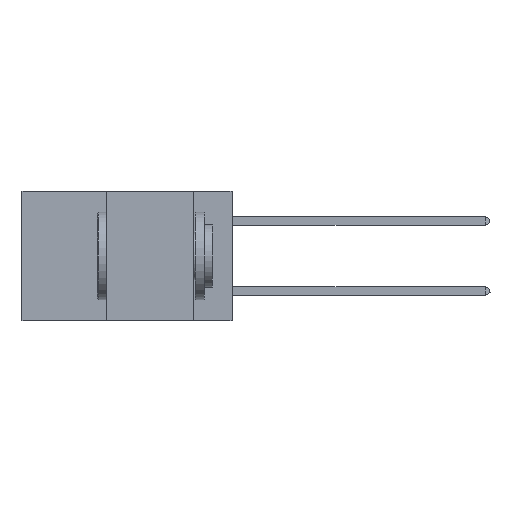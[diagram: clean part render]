
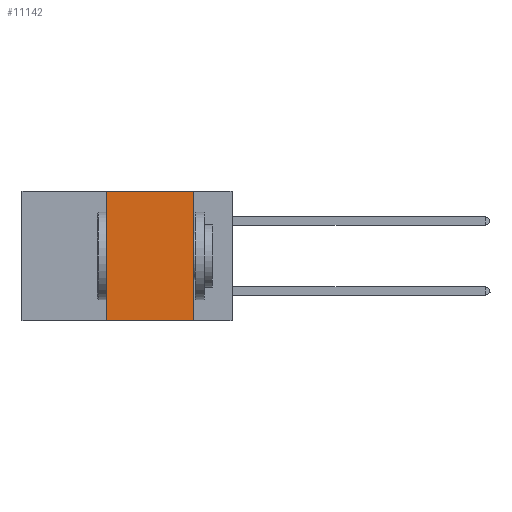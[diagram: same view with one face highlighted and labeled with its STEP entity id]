
A CAD part, left-side view. The second image highlights one B-rep face of the part: STEP entity #11142.
In plain terms, the highlighted planar face has unit normal (-1, 0, 0).
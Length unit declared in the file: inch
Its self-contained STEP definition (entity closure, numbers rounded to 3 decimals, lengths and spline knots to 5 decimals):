
#595 = CARTESIAN_POINT ( 'NONE',  ( 0., 0.6, -0.37 ) ) ;
#807 = VECTOR ( 'NONE', #4063, 39.37008 ) ;
#1679 = DIRECTION ( 'NONE',  ( 0., -1., 0. ) ) ;
#1815 = DIRECTION ( 'NONE',  ( 0., 0., -1. ) ) ;
#2269 = DIRECTION ( 'NONE',  ( 0., -1., 0. ) ) ;
#3034 = LINE ( 'NONE', #10944, #12753 ) ;
#3275 = EDGE_CURVE ( 'NONE', #13437, #11433, #10477, .T. ) ;
#4063 = DIRECTION ( 'NONE',  ( 0., 0., -1. ) ) ;
#4498 = FACE_OUTER_BOUND ( 'NONE', #11702, .T. ) ;
#4716 = ORIENTED_EDGE ( 'NONE', *, *, #8794, .T. ) ;
#4725 = VECTOR ( 'NONE', #1679, 39.37008 ) ;
#5052 = VERTEX_POINT ( 'NONE', #6766 ) ;
#6230 = AXIS2_PLACEMENT_3D ( 'NONE', #10564, #11610, #1815 ) ;
#6529 = ORIENTED_EDGE ( 'NONE', *, *, #3275, .F. ) ;
#6677 = DIRECTION ( 'NONE',  ( 0., 0., 1. ) ) ;
#6766 = CARTESIAN_POINT ( 'NONE',  ( 0., 0.36, 0. ) ) ;
#7345 = EDGE_CURVE ( 'NONE', #12144, #5052, #3034, .T. ) ;
#7380 = PLANE ( 'NONE',  #6230 ) ;
#7540 = EDGE_CURVE ( 'NONE', #5052, #13437, #13109, .T. ) ;
#7649 = CARTESIAN_POINT ( 'NONE',  ( 0., 0.6, 0. ) ) ;
#7983 = ORIENTED_EDGE ( 'NONE', *, *, #7540, .F. ) ;
#8764 = ORIENTED_EDGE ( 'NONE', *, *, #7345, .F. ) ;
#8794 = EDGE_CURVE ( 'NONE', #12144, #11433, #10504, .T. ) ;
#9656 = CARTESIAN_POINT ( 'NONE',  ( 0., 0.11, -0.37 ) ) ;
#10169 = VECTOR ( 'NONE', #2269, 39.37008 ) ;
#10222 = CARTESIAN_POINT ( 'NONE',  ( 0., 0.36, -0.37 ) ) ;
#10477 = LINE ( 'NONE', #11463, #807 ) ;
#10504 = LINE ( 'NONE', #595, #4725 ) ;
#10564 = CARTESIAN_POINT ( 'NONE',  ( 0., 0.6, 0. ) ) ;
#10944 = CARTESIAN_POINT ( 'NONE',  ( 0., 0.36, 0. ) ) ;
#11142 = ADVANCED_FACE ( 'NONE', ( #4498 ), #7380, .F. ) ;
#11433 = VERTEX_POINT ( 'NONE', #9656 ) ;
#11463 = CARTESIAN_POINT ( 'NONE',  ( 0., 0.11, 0. ) ) ;
#11610 = DIRECTION ( 'NONE',  ( 1., 0., 0. ) ) ;
#11702 = EDGE_LOOP ( 'NONE', ( #6529, #7983, #8764, #4716 ) ) ;
#12144 = VERTEX_POINT ( 'NONE', #10222 ) ;
#12753 = VECTOR ( 'NONE', #6677, 39.37008 ) ;
#13109 = LINE ( 'NONE', #7649, #10169 ) ;
#13437 = VERTEX_POINT ( 'NONE', #13961 ) ;
#13961 = CARTESIAN_POINT ( 'NONE',  ( 0., 0.11, 0. ) ) ;
